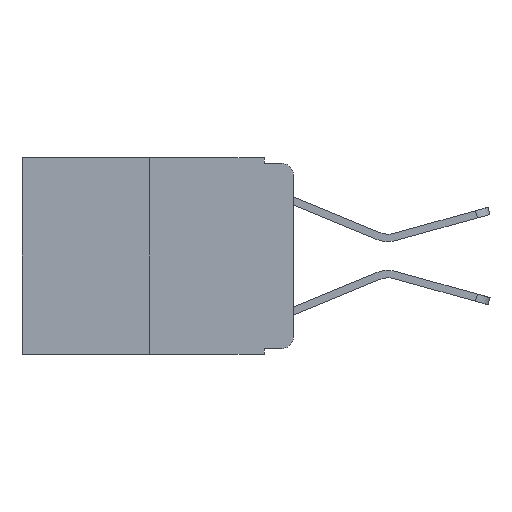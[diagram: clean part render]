
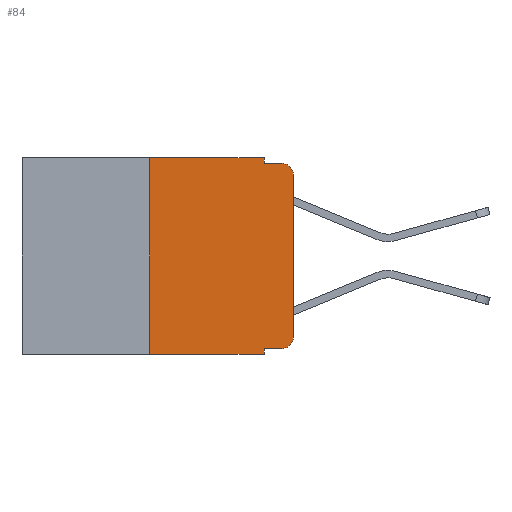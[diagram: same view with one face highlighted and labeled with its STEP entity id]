
A CAD part, left-side view. The second image highlights one B-rep face of the part: STEP entity #84.
In plain terms, the highlighted planar face has unit normal (-1, 0, 0).
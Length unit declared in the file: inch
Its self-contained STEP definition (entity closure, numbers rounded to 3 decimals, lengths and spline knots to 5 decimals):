
#23 = DIRECTION ( 'NONE',  ( 0., -1., 0. ) ) ;
#84 = ADVANCED_FACE ( 'NONE', ( #7741 ), #441, .F. ) ;
#100 = EDGE_CURVE ( 'NONE', #706, #6710, #5590, .T. ) ;
#194 = CARTESIAN_POINT ( 'NONE',  ( 0., 0.25, 0. ) ) ;
#255 = VERTEX_POINT ( 'NONE', #9620 ) ;
#441 = PLANE ( 'NONE',  #8217 ) ;
#525 = EDGE_CURVE ( 'NONE', #706, #1859, #2981, .T. ) ;
#619 = CARTESIAN_POINT ( 'NONE',  ( 0., 0.02, -0.313 ) ) ;
#706 = VERTEX_POINT ( 'NONE', #3254 ) ;
#768 = VECTOR ( 'NONE', #935, 39.37008 ) ;
#836 = CARTESIAN_POINT ( 'NONE',  ( 0., 0.051, -0.01 ) ) ;
#935 = DIRECTION ( 'NONE',  ( 0., -1., 0. ) ) ;
#1089 = CARTESIAN_POINT ( 'NONE',  ( 0., 0.051, 0. ) ) ;
#1219 = DIRECTION ( 'NONE',  ( 0., -1., 0. ) ) ;
#1317 = DIRECTION ( 'NONE',  ( 1., 0., 0. ) ) ;
#1337 = LINE ( 'NONE', #836, #8032 ) ;
#1341 = CARTESIAN_POINT ( 'NONE',  ( 0., 0.051, -0.333 ) ) ;
#1378 = DIRECTION ( 'NONE',  ( 0., 0., -1. ) ) ;
#1529 = ORIENTED_EDGE ( 'NONE', *, *, #10136, .F. ) ;
#1725 = CARTESIAN_POINT ( 'NONE',  ( 0., 0.473, -0.343 ) ) ;
#1765 = DIRECTION ( 'NONE',  ( 0., 0., 1. ) ) ;
#1804 = ORIENTED_EDGE ( 'NONE', *, *, #9342, .F. ) ;
#1859 = VERTEX_POINT ( 'NONE', #10419 ) ;
#1898 = VERTEX_POINT ( 'NONE', #3858 ) ;
#2020 = ORIENTED_EDGE ( 'NONE', *, *, #7333, .F. ) ;
#2140 = VECTOR ( 'NONE', #4770, 39.37008 ) ;
#2154 = DIRECTION ( 'NONE',  ( 0., 0., -1. ) ) ;
#2522 = AXIS2_PLACEMENT_3D ( 'NONE', #5055, #5130, #5163 ) ;
#2594 = ORIENTED_EDGE ( 'NONE', *, *, #9934, .T. ) ;
#2657 = CARTESIAN_POINT ( 'NONE',  ( 0., 0.051, 0. ) ) ;
#2721 = CARTESIAN_POINT ( 'NONE',  ( 0., 0., -0.313 ) ) ;
#2893 = LINE ( 'NONE', #6193, #6506 ) ;
#2981 = LINE ( 'NONE', #1341, #8607 ) ;
#3102 = EDGE_CURVE ( 'NONE', #4354, #255, #5144, .T. ) ;
#3122 = ORIENTED_EDGE ( 'NONE', *, *, #3102, .F. ) ;
#3254 = CARTESIAN_POINT ( 'NONE',  ( 0., 0.051, -0.333 ) ) ;
#3858 = CARTESIAN_POINT ( 'NONE',  ( 0., 0.02, -0.01 ) ) ;
#3920 = ORIENTED_EDGE ( 'NONE', *, *, #100, .F. ) ;
#3950 = DIRECTION ( 'NONE',  ( 0., -1., 0. ) ) ;
#4088 = CARTESIAN_POINT ( 'NONE',  ( 0., 0.051, -0.01 ) ) ;
#4354 = VERTEX_POINT ( 'NONE', #5425 ) ;
#4594 = DIRECTION ( 'NONE',  ( 0., 0., -1. ) ) ;
#4634 = CARTESIAN_POINT ( 'NONE',  ( 0., 0.051, 0. ) ) ;
#4770 = DIRECTION ( 'NONE',  ( 0., 0., -1. ) ) ;
#5009 = CARTESIAN_POINT ( 'NONE',  ( 0., 0.051, -0.343 ) ) ;
#5055 = CARTESIAN_POINT ( 'NONE',  ( 0., 0.02, -0.03 ) ) ;
#5130 = DIRECTION ( 'NONE',  ( -1., 0., 0. ) ) ;
#5144 = LINE ( 'NONE', #194, #6292 ) ;
#5163 = DIRECTION ( 'NONE',  ( 0., 0., -1. ) ) ;
#5330 = VECTOR ( 'NONE', #4594, 39.37008 ) ;
#5425 = CARTESIAN_POINT ( 'NONE',  ( 0., 0.25, -0.343 ) ) ;
#5564 = DIRECTION ( 'NONE',  ( -1., 0., 0. ) ) ;
#5590 = LINE ( 'NONE', #4634, #5330 ) ;
#6193 = CARTESIAN_POINT ( 'NONE',  ( 0., 0.473, 0. ) ) ;
#6276 = EDGE_CURVE ( 'NONE', #4354, #6710, #10143, .T. ) ;
#6286 = ORIENTED_EDGE ( 'NONE', *, *, #6852, .T. ) ;
#6292 = VECTOR ( 'NONE', #8311, 39.37008 ) ;
#6318 = CIRCLE ( 'NONE', #7105, 0.02 ) ;
#6356 = VERTEX_POINT ( 'NONE', #2721 ) ;
#6506 = VECTOR ( 'NONE', #1219, 39.37008 ) ;
#6644 = ORIENTED_EDGE ( 'NONE', *, *, #525, .T. ) ;
#6710 = VERTEX_POINT ( 'NONE', #5009 ) ;
#6852 = EDGE_CURVE ( 'NONE', #1859, #6356, #6318, .T. ) ;
#6899 = VECTOR ( 'NONE', #1765, 39.37008 ) ;
#7105 = AXIS2_PLACEMENT_3D ( 'NONE', #619, #5564, #1378 ) ;
#7149 = LINE ( 'NONE', #8278, #6899 ) ;
#7185 = ORIENTED_EDGE ( 'NONE', *, *, #9883, .T. ) ;
#7333 = EDGE_CURVE ( 'NONE', #9973, #9320, #9233, .T. ) ;
#7741 = FACE_OUTER_BOUND ( 'NONE', #8168, .T. ) ;
#8032 = VECTOR ( 'NONE', #23, 39.37008 ) ;
#8168 = EDGE_LOOP ( 'NONE', ( #2594, #7185, #1804, #2020, #1529, #3122, #9734, #3920, #6644, #6286 ) ) ;
#8217 = AXIS2_PLACEMENT_3D ( 'NONE', #8692, #1317, #2154 ) ;
#8278 = CARTESIAN_POINT ( 'NONE',  ( 0., 0., 0. ) ) ;
#8311 = DIRECTION ( 'NONE',  ( 0., 0., 1. ) ) ;
#8607 = VECTOR ( 'NONE', #3950, 39.37008 ) ;
#8692 = CARTESIAN_POINT ( 'NONE',  ( 0., 0.473, 0. ) ) ;
#8790 = CIRCLE ( 'NONE', #2522, 0.02 ) ;
#9233 = LINE ( 'NONE', #1089, #2140 ) ;
#9320 = VERTEX_POINT ( 'NONE', #4088 ) ;
#9342 = EDGE_CURVE ( 'NONE', #9320, #1898, #1337, .T. ) ;
#9387 = CARTESIAN_POINT ( 'NONE',  ( 0., 0., -0.03 ) ) ;
#9620 = CARTESIAN_POINT ( 'NONE',  ( 0., 0.25, 0. ) ) ;
#9734 = ORIENTED_EDGE ( 'NONE', *, *, #6276, .T. ) ;
#9883 = EDGE_CURVE ( 'NONE', #10111, #1898, #8790, .T. ) ;
#9934 = EDGE_CURVE ( 'NONE', #6356, #10111, #7149, .T. ) ;
#9973 = VERTEX_POINT ( 'NONE', #2657 ) ;
#10111 = VERTEX_POINT ( 'NONE', #9387 ) ;
#10136 = EDGE_CURVE ( 'NONE', #255, #9973, #2893, .T. ) ;
#10143 = LINE ( 'NONE', #1725, #768 ) ;
#10419 = CARTESIAN_POINT ( 'NONE',  ( 0., 0.02, -0.333 ) ) ;
